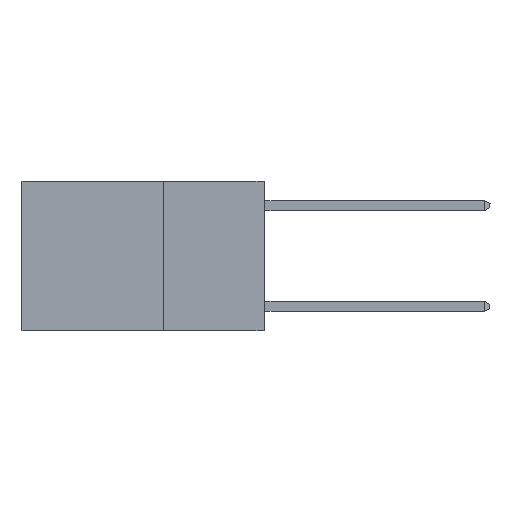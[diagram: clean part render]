
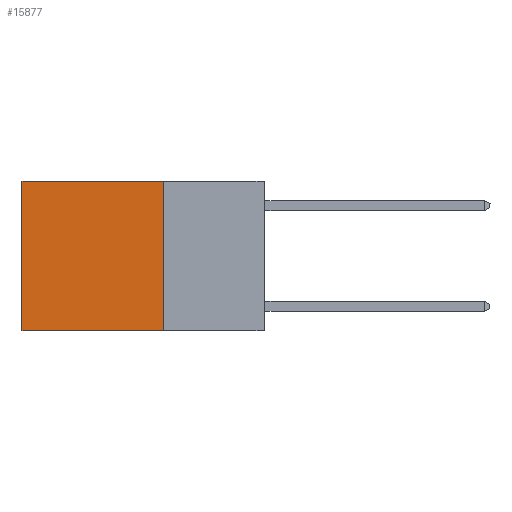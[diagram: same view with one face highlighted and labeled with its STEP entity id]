
A CAD part, left-side view. The second image highlights one B-rep face of the part: STEP entity #15877.
In plain terms, the highlighted planar face has unit normal (-1, 0, 0).
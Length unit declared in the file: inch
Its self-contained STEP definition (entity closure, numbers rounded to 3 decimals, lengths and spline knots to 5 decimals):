
#101 = ORIENTED_EDGE ( 'NONE', *, *, #4738, .T. ) ;
#223 = DIRECTION ( 'NONE',  ( 0., 0., -1. ) ) ;
#1946 = LINE ( 'NONE', #16647, #8795 ) ;
#2188 = DIRECTION ( 'NONE',  ( 0., 0., -1. ) ) ;
#2295 = CARTESIAN_POINT ( 'NONE',  ( 0.2625, 0.25, -0.37 ) ) ;
#2360 = CARTESIAN_POINT ( 'NONE',  ( 0.2625, 0.25, 0. ) ) ;
#2924 = CARTESIAN_POINT ( 'NONE',  ( 0.2625, 0.25, 0. ) ) ;
#2941 = VERTEX_POINT ( 'NONE', #15780 ) ;
#3005 = CARTESIAN_POINT ( 'NONE',  ( 0.2625, 0.6, -0.37 ) ) ;
#3635 = LINE ( 'NONE', #2360, #6868 ) ;
#3690 = DIRECTION ( 'NONE',  ( 0., 1., 0. ) ) ;
#3753 = DIRECTION ( 'NONE',  ( 0., 1., 0. ) ) ;
#3889 = CARTESIAN_POINT ( 'NONE',  ( 0.2625, 0.25, 0. ) ) ;
#4004 = ORIENTED_EDGE ( 'NONE', *, *, #11394, .F. ) ;
#4738 = EDGE_CURVE ( 'NONE', #11131, #5428, #1946, .T. ) ;
#5316 = AXIS2_PLACEMENT_3D ( 'NONE', #2924, #15192, #7070 ) ;
#5428 = VERTEX_POINT ( 'NONE', #3005 ) ;
#5695 = PLANE ( 'NONE',  #5316 ) ;
#6801 = LINE ( 'NONE', #13150, #13590 ) ;
#6850 = ORIENTED_EDGE ( 'NONE', *, *, #9092, .T. ) ;
#6868 = VECTOR ( 'NONE', #3753, 39.37008 ) ;
#7070 = DIRECTION ( 'NONE',  ( 0., 0., -1. ) ) ;
#7206 = CARTESIAN_POINT ( 'NONE',  ( 0.2625, 0.6, 0. ) ) ;
#7756 = EDGE_LOOP ( 'NONE', ( #101, #14167, #4004, #6850 ) ) ;
#8085 = VECTOR ( 'NONE', #3690, 39.37008 ) ;
#8597 = VERTEX_POINT ( 'NONE', #3889 ) ;
#8795 = VECTOR ( 'NONE', #223, 39.37008 ) ;
#8939 = LINE ( 'NONE', #2295, #8085 ) ;
#9092 = EDGE_CURVE ( 'NONE', #8597, #11131, #3635, .T. ) ;
#11131 = VERTEX_POINT ( 'NONE', #7206 ) ;
#11394 = EDGE_CURVE ( 'NONE', #8597, #2941, #6801, .T. ) ;
#13150 = CARTESIAN_POINT ( 'NONE',  ( 0.2625, 0.25, 0. ) ) ;
#13590 = VECTOR ( 'NONE', #2188, 39.37008 ) ;
#14167 = ORIENTED_EDGE ( 'NONE', *, *, #16139, .F. ) ;
#15192 = DIRECTION ( 'NONE',  ( 1., 0., 0. ) ) ;
#15780 = CARTESIAN_POINT ( 'NONE',  ( 0.2625, 0.25, -0.37 ) ) ;
#15877 = ADVANCED_FACE ( 'NONE', ( #15965 ), #5695, .F. ) ;
#15965 = FACE_OUTER_BOUND ( 'NONE', #7756, .T. ) ;
#16139 = EDGE_CURVE ( 'NONE', #2941, #5428, #8939, .T. ) ;
#16647 = CARTESIAN_POINT ( 'NONE',  ( 0.2625, 0.6, 0. ) ) ;
